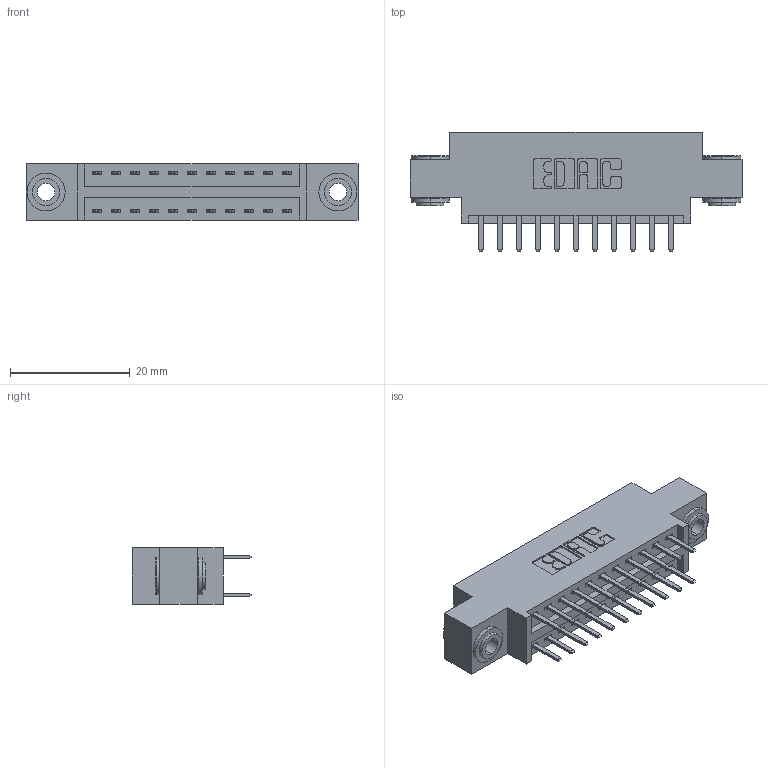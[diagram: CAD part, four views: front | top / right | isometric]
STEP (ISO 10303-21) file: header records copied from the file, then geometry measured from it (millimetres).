
FILE_DESCRIPTION (( 'STEP AP203' ), '1' );
FILE_NAME ('396-022-520-803.STEP', '2018-09-01T08:36:44', ( '' ), ( '' ), 'SwSTEP 2.0', 'SolidWorks 2016', '' );
FILE_SCHEMA (( 'CONFIG_CONTROL_DESIGN' ));
Length unit declared in the file: inch
Products named in the file (4): 346 Part_0.170 Offset - 0.156 Dia-TH; 345-292-001_345-293-120; 345-250-002_345-250-002-102; 396-022-520-803
Assembly tree (25 placements, depth 2):
  396-022-520-803
    346 Part_0.170 Offset - 0.156 Dia-TH
    345-292-001_345-293-120  x22
    345-250-002_345-250-002-102  x2
Bounding box: 55.5 x 20.02 x 9.4 mm (x, y, z)
Volume: 5026.2 mm3; surface area: 6792.7 mm2
Topology: 25 solids, 25 shells, 1396 faces, 4003 edges, 2606 vertices
Faces by surface type: plane 904, cylinder 484, cone 8
Entity records: 12248 total; most frequent: CARTESIAN_POINT 2051, ORIENTED_EDGE 1966, DIRECTION 1877, EDGE_CURVE 983, LINE 779, VECTOR 779, VERTEX_POINT 650, AXIS2_PLACEMENT_3D 549
